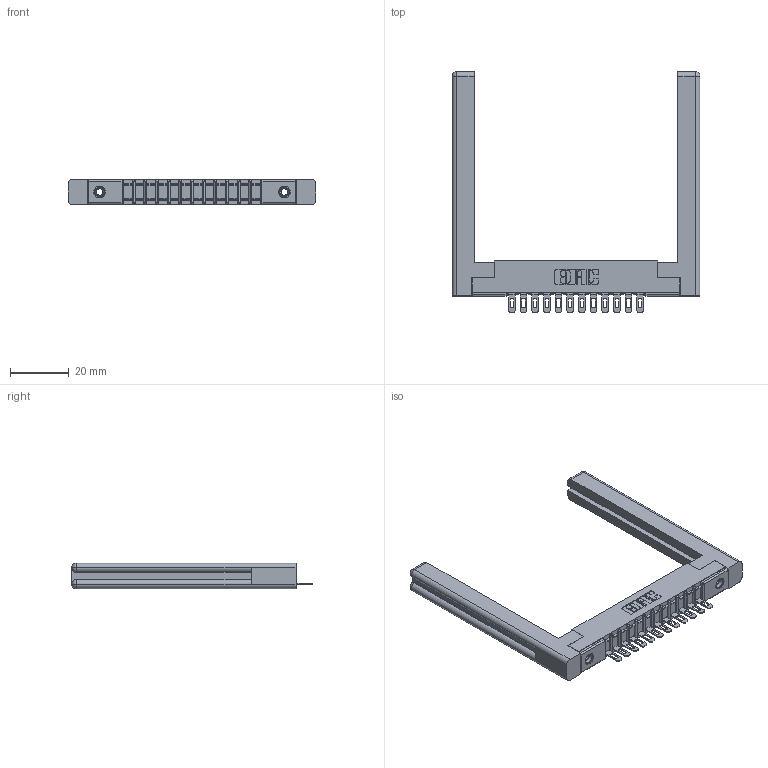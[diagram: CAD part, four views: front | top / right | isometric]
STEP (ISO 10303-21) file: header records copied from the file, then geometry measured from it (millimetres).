
FILE_DESCRIPTION (( 'STEP AP203' ), '1' );
FILE_NAME ('357-012-501-158.STEP', '2019-09-16T19:06:39', ( '' ), ( '' ), 'SwSTEP 2.0', 'SolidWorks 2016', '' );
FILE_SCHEMA (( 'CONFIG_CONTROL_DESIGN' ));
Length unit declared in the file: inch
Products named in the file (5): 345-250-001_345-250-001-102; 307-290-002_501; 307 Part_.156 Dia Mounting Holes; 307-220-058; 357-012-501-158
Assembly tree (17 placements, depth 2):
  357-012-501-158
    307 Part_.156 Dia Mounting Holes
    307-290-002_501  x12
    307-220-058  x2
    345-250-001_345-250-001-102  x2
Bounding box: 84.18 x 81.74 x 8.71 mm (x, y, z)
Volume: 13240.7 mm3; surface area: 14666 mm2
Topology: 17 solids, 17 shells, 1185 faces, 3533 edges, 2306 vertices
Faces by surface type: plane 682, cylinder 453, sphere 26, torus 12, cone 12
Entity records: 17413 total; most frequent: CARTESIAN_POINT 2939, ORIENTED_EDGE 2868, DIRECTION 2834, EDGE_CURVE 1434, LINE 1076, VECTOR 1076, VERTEX_POINT 930, AXIS2_PLACEMENT_3D 879
